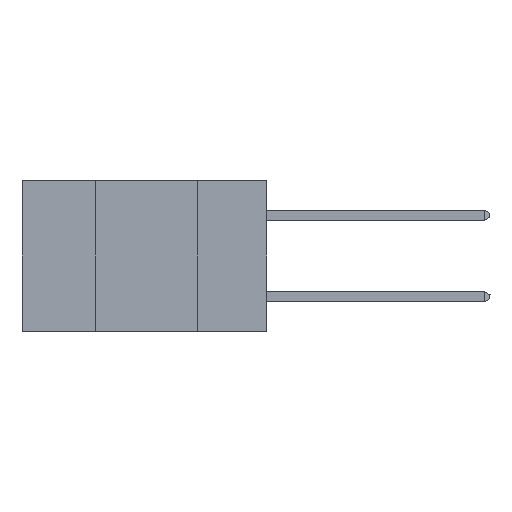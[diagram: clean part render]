
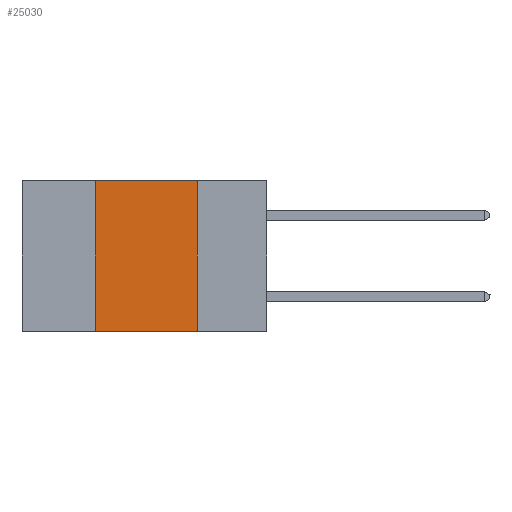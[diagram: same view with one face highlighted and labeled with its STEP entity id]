
A CAD part, left-side view. The second image highlights one B-rep face of the part: STEP entity #25030.
In plain terms, the highlighted planar face has unit normal (-1, 0, 0).
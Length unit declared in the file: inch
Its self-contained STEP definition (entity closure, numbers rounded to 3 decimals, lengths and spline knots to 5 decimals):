
#291 = LINE ( 'NONE', #19649, #6006 ) ;
#738 = CARTESIAN_POINT ( 'NONE',  ( 0., 0.6, -0.37 ) ) ;
#944 = VERTEX_POINT ( 'NONE', #17040 ) ;
#1181 = LINE ( 'NONE', #738, #20073 ) ;
#1821 = CARTESIAN_POINT ( 'NONE',  ( 0., 0.42, -0.37 ) ) ;
#4806 = CARTESIAN_POINT ( 'NONE',  ( 0., 0.17, 0. ) ) ;
#5244 = ORIENTED_EDGE ( 'NONE', *, *, #10419, .T. ) ;
#5710 = EDGE_LOOP ( 'NONE', ( #35782, #27814, #12019, #5244 ) ) ;
#6006 = VECTOR ( 'NONE', #31203, 39.37008 ) ;
#6370 = CARTESIAN_POINT ( 'NONE',  ( 0., 0.17, 0. ) ) ;
#6562 = CARTESIAN_POINT ( 'NONE',  ( 0., 0.6, 0. ) ) ;
#8521 = EDGE_CURVE ( 'NONE', #29934, #22922, #31968, .T. ) ;
#10419 = EDGE_CURVE ( 'NONE', #29176, #944, #1181, .T. ) ;
#12019 = ORIENTED_EDGE ( 'NONE', *, *, #24132, .F. ) ;
#12127 = CARTESIAN_POINT ( 'NONE',  ( 0., 0.6, 0. ) ) ;
#12489 = DIRECTION ( 'NONE',  ( 1., 0., 0. ) ) ;
#15590 = DIRECTION ( 'NONE',  ( 0., -1., 0. ) ) ;
#17040 = CARTESIAN_POINT ( 'NONE',  ( 0., 0.17, -0.37 ) ) ;
#18653 = FACE_OUTER_BOUND ( 'NONE', #5710, .T. ) ;
#19649 = CARTESIAN_POINT ( 'NONE',  ( 0., 0.42, 0. ) ) ;
#20073 = VECTOR ( 'NONE', #15590, 39.37008 ) ;
#22922 = VERTEX_POINT ( 'NONE', #4806 ) ;
#23568 = DIRECTION ( 'NONE',  ( 0., 0., -1. ) ) ;
#23600 = AXIS2_PLACEMENT_3D ( 'NONE', #12127, #12489, #23568 ) ;
#24132 = EDGE_CURVE ( 'NONE', #29176, #29934, #291, .T. ) ;
#25030 = ADVANCED_FACE ( 'NONE', ( #18653 ), #29329, .F. ) ;
#26016 = DIRECTION ( 'NONE',  ( 0., 0., -1. ) ) ;
#26937 = EDGE_CURVE ( 'NONE', #22922, #944, #29942, .T. ) ;
#27814 = ORIENTED_EDGE ( 'NONE', *, *, #8521, .F. ) ;
#29040 = DIRECTION ( 'NONE',  ( 0., -1., 0. ) ) ;
#29176 = VERTEX_POINT ( 'NONE', #1821 ) ;
#29329 = PLANE ( 'NONE',  #23600 ) ;
#29934 = VERTEX_POINT ( 'NONE', #31115 ) ;
#29942 = LINE ( 'NONE', #6370, #33030 ) ;
#31115 = CARTESIAN_POINT ( 'NONE',  ( 0., 0.42, 0. ) ) ;
#31203 = DIRECTION ( 'NONE',  ( 0., 0., 1. ) ) ;
#31968 = LINE ( 'NONE', #6562, #34159 ) ;
#33030 = VECTOR ( 'NONE', #26016, 39.37008 ) ;
#34159 = VECTOR ( 'NONE', #29040, 39.37008 ) ;
#35782 = ORIENTED_EDGE ( 'NONE', *, *, #26937, .F. ) ;
